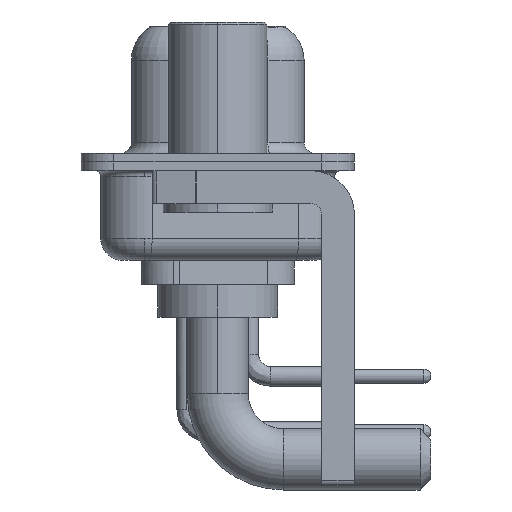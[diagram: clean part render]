
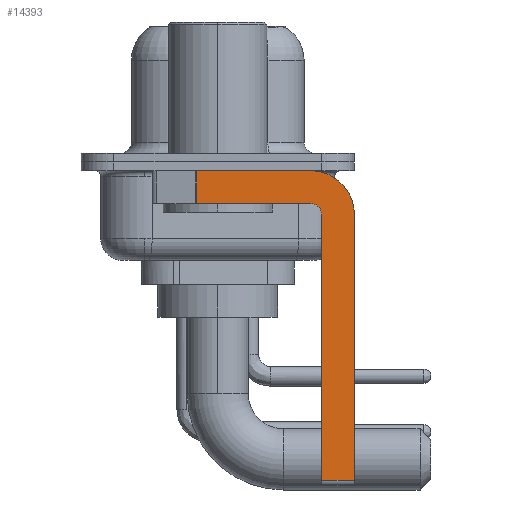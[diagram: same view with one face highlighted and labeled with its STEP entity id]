
A CAD part, left-side view. The second image highlights one B-rep face of the part: STEP entity #14393.
In plain terms, the highlighted planar face has unit normal (-1, 0, 0).
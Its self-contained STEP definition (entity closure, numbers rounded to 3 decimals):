
#537 = ORIENTED_EDGE ( 'NONE', *, *, #2837, .F. ) ;
#612 = VECTOR ( 'NONE', #3582, 1000. ) ;
#1173 = CARTESIAN_POINT ( 'NONE',  ( -2.9, -4.75, -2.4 ) ) ;
#1461 = ORIENTED_EDGE ( 'NONE', *, *, #11969, .F. ) ;
#1588 = LINE ( 'NONE', #3107, #20921 ) ;
#2641 = ORIENTED_EDGE ( 'NONE', *, *, #9926, .T. ) ;
#2837 = EDGE_CURVE ( 'NONE', #17869, #6806, #15328, .T. ) ;
#2937 = VERTEX_POINT ( 'NONE', #6687 ) ;
#3045 = DIRECTION ( 'NONE',  ( 1., 0., 0. ) ) ;
#3107 = CARTESIAN_POINT ( 'NONE',  ( -2.9, -4.25, -14.55 ) ) ;
#3263 = CARTESIAN_POINT ( 'NONE',  ( -2.9, 0.978, -1.9 ) ) ;
#3280 = VERTEX_POINT ( 'NONE', #16232 ) ;
#3543 = DIRECTION ( 'NONE',  ( 0., 0., -1. ) ) ;
#3582 = DIRECTION ( 'NONE',  ( 0., 0., -1. ) ) ;
#4122 = DIRECTION ( 'NONE',  ( 0., 0., 1. ) ) ;
#4381 = DIRECTION ( 'NONE',  ( 0., 0., 1. ) ) ;
#4911 = CARTESIAN_POINT ( 'NONE',  ( -2.9, -4.25, -0.4 ) ) ;
#5187 = PLANE ( 'NONE',  #16122 ) ;
#5244 = AXIS2_PLACEMENT_3D ( 'NONE', #6029, #19331, #4381 ) ;
#5825 = EDGE_CURVE ( 'NONE', #2937, #21346, #6877, .T. ) ;
#5833 = DIRECTION ( 'NONE',  ( 0., 0., -1. ) ) ;
#6029 = CARTESIAN_POINT ( 'NONE',  ( -2.9, -4.25, -2.4 ) ) ;
#6078 = LINE ( 'NONE', #10957, #17397 ) ;
#6244 = CARTESIAN_POINT ( 'NONE',  ( -2.9, 0.978, -1.9 ) ) ;
#6332 = LINE ( 'NONE', #13191, #13657 ) ;
#6687 = CARTESIAN_POINT ( 'NONE',  ( -2.9, 0.978, -0.4 ) ) ;
#6806 = VERTEX_POINT ( 'NONE', #9759 ) ;
#6877 = LINE ( 'NONE', #3263, #612 ) ;
#7587 = DIRECTION ( 'NONE',  ( 0., -1., 0. ) ) ;
#8223 = ORIENTED_EDGE ( 'NONE', *, *, #17443, .F. ) ;
#8290 = CARTESIAN_POINT ( 'NONE',  ( -2.9, -4.25, -2.4 ) ) ;
#8323 = EDGE_CURVE ( 'NONE', #2937, #17410, #6078, .T. ) ;
#8998 = CARTESIAN_POINT ( 'NONE',  ( -2.9, -6.25, -2.4 ) ) ;
#9352 = ORIENTED_EDGE ( 'NONE', *, *, #20023, .F. ) ;
#9759 = CARTESIAN_POINT ( 'NONE',  ( -2.9, -4.25, -1.9 ) ) ;
#9909 = DIRECTION ( 'NONE',  ( 0., 0., -1. ) ) ;
#9926 = EDGE_CURVE ( 'NONE', #3280, #11302, #1588, .T. ) ;
#10308 = FACE_OUTER_BOUND ( 'NONE', #17065, .T. ) ;
#10957 = CARTESIAN_POINT ( 'NONE',  ( -2.9, 3., -0.4 ) ) ;
#11302 = VERTEX_POINT ( 'NONE', #19565 ) ;
#11724 = CARTESIAN_POINT ( 'NONE',  ( -2.9, -4.25, -2.4 ) ) ;
#11827 = DIRECTION ( 'NONE',  ( 1., 0., 0. ) ) ;
#11969 = EDGE_CURVE ( 'NONE', #3280, #17869, #12086, .T. ) ;
#12086 = LINE ( 'NONE', #19079, #19587 ) ;
#12389 = CARTESIAN_POINT ( 'NONE',  ( -2.9, -6.25, -2.4 ) ) ;
#12485 = CIRCLE ( 'NONE', #14237, 2. ) ;
#12656 = VERTEX_POINT ( 'NONE', #12389 ) ;
#12813 = DIRECTION ( 'NONE',  ( 0., -1., 0. ) ) ;
#13191 = CARTESIAN_POINT ( 'NONE',  ( -2.9, -4.25, -1.9 ) ) ;
#13657 = VECTOR ( 'NONE', #17887, 1000. ) ;
#14237 = AXIS2_PLACEMENT_3D ( 'NONE', #8290, #3045, #9909 ) ;
#14393 = ADVANCED_FACE ( 'NONE', ( #10308 ), #5187, .F. ) ;
#15213 = ORIENTED_EDGE ( 'NONE', *, *, #5825, .T. ) ;
#15219 = ORIENTED_EDGE ( 'NONE', *, *, #8323, .F. ) ;
#15328 = CIRCLE ( 'NONE', #5244, 0.5 ) ;
#15893 = EDGE_CURVE ( 'NONE', #12656, #11302, #20877, .T. ) ;
#16122 = AXIS2_PLACEMENT_3D ( 'NONE', #11724, #11827, #3543 ) ;
#16232 = CARTESIAN_POINT ( 'NONE',  ( -2.9, -4.75, -14.55 ) ) ;
#17065 = EDGE_LOOP ( 'NONE', ( #15219, #15213, #9352, #537, #1461, #2641, #19406, #8223 ) ) ;
#17263 = VECTOR ( 'NONE', #5833, 1000. ) ;
#17397 = VECTOR ( 'NONE', #7587, 1000. ) ;
#17410 = VERTEX_POINT ( 'NONE', #4911 ) ;
#17443 = EDGE_CURVE ( 'NONE', #17410, #12656, #12485, .T. ) ;
#17869 = VERTEX_POINT ( 'NONE', #1173 ) ;
#17887 = DIRECTION ( 'NONE',  ( 0., 1., 0. ) ) ;
#19079 = CARTESIAN_POINT ( 'NONE',  ( -2.9, -4.75, -14.8 ) ) ;
#19331 = DIRECTION ( 'NONE',  ( -1., 0., 0. ) ) ;
#19406 = ORIENTED_EDGE ( 'NONE', *, *, #15893, .F. ) ;
#19565 = CARTESIAN_POINT ( 'NONE',  ( -2.9, -6.25, -14.55 ) ) ;
#19587 = VECTOR ( 'NONE', #4122, 1000. ) ;
#20023 = EDGE_CURVE ( 'NONE', #6806, #21346, #6332, .T. ) ;
#20877 = LINE ( 'NONE', #8998, #17263 ) ;
#20921 = VECTOR ( 'NONE', #12813, 1000. ) ;
#21346 = VERTEX_POINT ( 'NONE', #6244 ) ;
